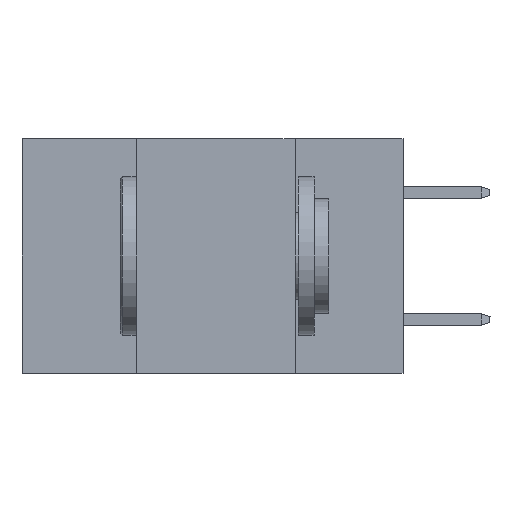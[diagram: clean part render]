
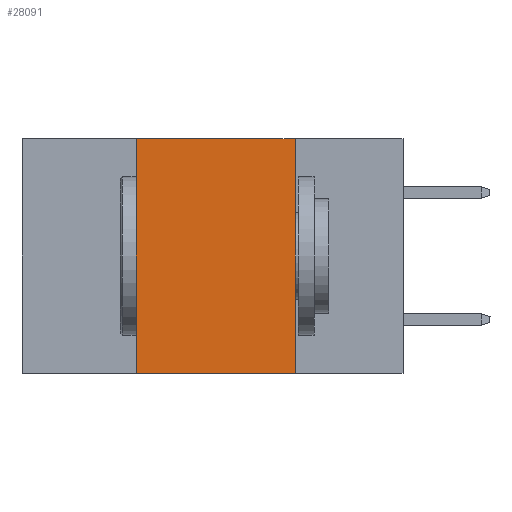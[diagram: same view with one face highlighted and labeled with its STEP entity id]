
A CAD part, left-side view. The second image highlights one B-rep face of the part: STEP entity #28091.
In plain terms, the highlighted planar face has unit normal (-1, 0, 0).
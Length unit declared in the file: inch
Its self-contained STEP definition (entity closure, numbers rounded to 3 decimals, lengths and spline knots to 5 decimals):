
#1306 = ORIENTED_EDGE ( 'NONE', *, *, #17499, .F. ) ;
#3964 = DIRECTION ( 'NONE',  ( 1., 0., 0. ) ) ;
#5385 = VECTOR ( 'NONE', #19227, 39.37008 ) ;
#5939 = EDGE_LOOP ( 'NONE', ( #27703, #1306, #26449, #25810 ) ) ;
#5961 = VERTEX_POINT ( 'NONE', #15459 ) ;
#6535 = DIRECTION ( 'NONE',  ( 0., 0., 1. ) ) ;
#6716 = VECTOR ( 'NONE', #18347, 39.37008 ) ;
#7297 = CARTESIAN_POINT ( 'NONE',  ( 0., 0.17, 0. ) ) ;
#8087 = CARTESIAN_POINT ( 'NONE',  ( 0., 0.42, 0. ) ) ;
#8669 = CARTESIAN_POINT ( 'NONE',  ( 0., 0.6, 0. ) ) ;
#9049 = CARTESIAN_POINT ( 'NONE',  ( 0., 0.6, 0. ) ) ;
#12482 = EDGE_CURVE ( 'NONE', #22113, #15299, #20778, .T. ) ;
#13245 = FACE_OUTER_BOUND ( 'NONE', #5939, .T. ) ;
#15299 = VERTEX_POINT ( 'NONE', #25417 ) ;
#15459 = CARTESIAN_POINT ( 'NONE',  ( 0., 0.42, -0.37 ) ) ;
#17499 = EDGE_CURVE ( 'NONE', #22042, #22113, #19567, .T. ) ;
#18211 = LINE ( 'NONE', #24496, #23925 ) ;
#18347 = DIRECTION ( 'NONE',  ( 0., -1., 0. ) ) ;
#18979 = DIRECTION ( 'NONE',  ( 0., 0., -1. ) ) ;
#19116 = AXIS2_PLACEMENT_3D ( 'NONE', #8669, #3964, #26313 ) ;
#19227 = DIRECTION ( 'NONE',  ( 0., -1., 0. ) ) ;
#19567 = LINE ( 'NONE', #9049, #6716 ) ;
#20051 = CARTESIAN_POINT ( 'NONE',  ( 0., 0.17, 0. ) ) ;
#20778 = LINE ( 'NONE', #7297, #21734 ) ;
#21330 = CARTESIAN_POINT ( 'NONE',  ( 0., 0.6, -0.37 ) ) ;
#21734 = VECTOR ( 'NONE', #18979, 39.37008 ) ;
#22042 = VERTEX_POINT ( 'NONE', #8087 ) ;
#22113 = VERTEX_POINT ( 'NONE', #20051 ) ;
#22665 = EDGE_CURVE ( 'NONE', #5961, #22042, #18211, .T. ) ;
#23925 = VECTOR ( 'NONE', #6535, 39.37008 ) ;
#24496 = CARTESIAN_POINT ( 'NONE',  ( 0., 0.42, 0. ) ) ;
#24541 = PLANE ( 'NONE',  #19116 ) ;
#25300 = EDGE_CURVE ( 'NONE', #5961, #15299, #26499, .T. ) ;
#25417 = CARTESIAN_POINT ( 'NONE',  ( 0., 0.17, -0.37 ) ) ;
#25810 = ORIENTED_EDGE ( 'NONE', *, *, #25300, .T. ) ;
#26313 = DIRECTION ( 'NONE',  ( 0., 0., -1. ) ) ;
#26449 = ORIENTED_EDGE ( 'NONE', *, *, #22665, .F. ) ;
#26499 = LINE ( 'NONE', #21330, #5385 ) ;
#27703 = ORIENTED_EDGE ( 'NONE', *, *, #12482, .F. ) ;
#28091 = ADVANCED_FACE ( 'NONE', ( #13245 ), #24541, .F. ) ;
